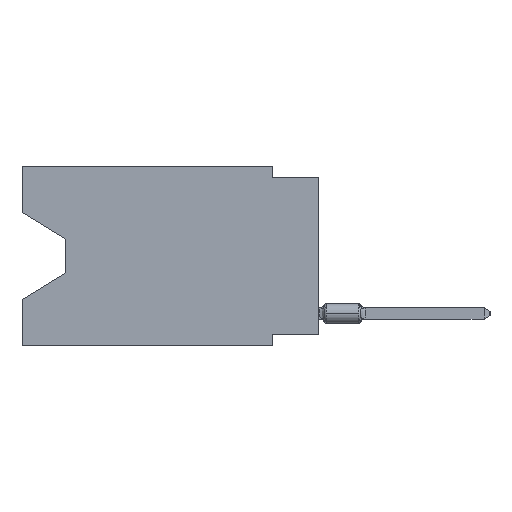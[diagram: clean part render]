
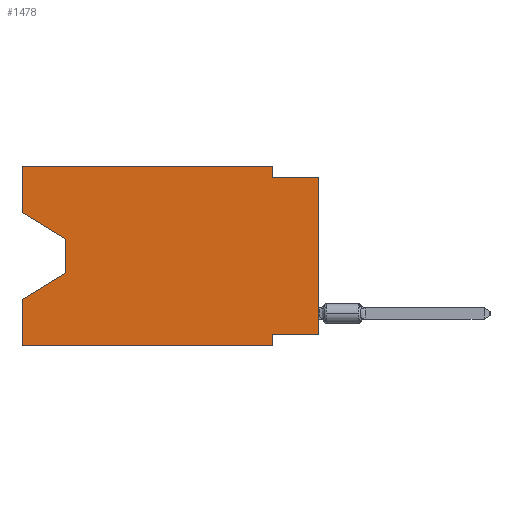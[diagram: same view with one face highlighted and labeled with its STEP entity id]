
A CAD part, left-side view. The second image highlights one B-rep face of the part: STEP entity #1478.
In plain terms, the highlighted planar face has unit normal (-1, 0, 0).
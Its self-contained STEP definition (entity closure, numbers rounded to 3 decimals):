
#391 = LINE ( 'NONE', #15423, #25079 ) ;
#925 = VERTEX_POINT ( 'NONE', #43220 ) ;
#1397 = CARTESIAN_POINT ( 'NONE',  ( 0., 16.383, -9.906 ) ) ;
#1478 = ADVANCED_FACE ( 'NONE', ( #54049 ), #12353, .F. ) ;
#2420 = DIRECTION ( 'NONE',  ( 1., 0., 0. ) ) ;
#3002 = DIRECTION ( 'NONE',  ( 0., 1., 0. ) ) ;
#3283 = VECTOR ( 'NONE', #44794, 1000. ) ;
#3491 = CARTESIAN_POINT ( 'NONE',  ( 0., 16.383, -9.906 ) ) ;
#3820 = LINE ( 'NONE', #13409, #64594 ) ;
#4241 = LINE ( 'NONE', #20308, #49185 ) ;
#4481 = VERTEX_POINT ( 'NONE', #1397 ) ;
#6366 = EDGE_CURVE ( 'NONE', #21469, #45907, #39562, .T. ) ;
#7596 = VERTEX_POINT ( 'NONE', #45051 ) ;
#8268 = AXIS2_PLACEMENT_3D ( 'NONE', #65319, #2420, #44143 ) ;
#8610 = VECTOR ( 'NONE', #54688, 1000. ) ;
#8970 = VECTOR ( 'NONE', #66699, 1000. ) ;
#8977 = EDGE_CURVE ( 'NONE', #925, #44547, #14672, .T. ) ;
#10274 = CARTESIAN_POINT ( 'NONE',  ( 0., 0., 0. ) ) ;
#11287 = LINE ( 'NONE', #10274, #15699 ) ;
#12353 = PLANE ( 'NONE',  #8268 ) ;
#13236 = VERTEX_POINT ( 'NONE', #47078 ) ;
#13409 = CARTESIAN_POINT ( 'NONE',  ( 0., 0., -0.635 ) ) ;
#14345 = CARTESIAN_POINT ( 'NONE',  ( 0., 13.97, -5.893 ) ) ;
#14672 = LINE ( 'NONE', #14345, #36406 ) ;
#14754 = CARTESIAN_POINT ( 'NONE',  ( 0., 13.97, -4.013 ) ) ;
#14878 = LINE ( 'NONE', #51452, #41210 ) ;
#15130 = ORIENTED_EDGE ( 'NONE', *, *, #55828, .T. ) ;
#15323 = ORIENTED_EDGE ( 'NONE', *, *, #56338, .F. ) ;
#15423 = CARTESIAN_POINT ( 'NONE',  ( 0., 13.97, -4.013 ) ) ;
#15699 = VECTOR ( 'NONE', #51976, 1000. ) ;
#16306 = VECTOR ( 'NONE', #29139, 1000. ) ;
#19307 = ORIENTED_EDGE ( 'NONE', *, *, #53118, .F. ) ;
#19395 = ORIENTED_EDGE ( 'NONE', *, *, #33960, .T. ) ;
#20308 = CARTESIAN_POINT ( 'NONE',  ( 0., 16.383, 0. ) ) ;
#20955 = ORIENTED_EDGE ( 'NONE', *, *, #58679, .F. ) ;
#21469 = VERTEX_POINT ( 'NONE', #47541 ) ;
#21693 = CARTESIAN_POINT ( 'NONE',  ( 0., 16.383, -7.36 ) ) ;
#22912 = CARTESIAN_POINT ( 'NONE',  ( 0., 16.383, 0. ) ) ;
#24276 = VERTEX_POINT ( 'NONE', #60544 ) ;
#25001 = LINE ( 'NONE', #3491, #16306 ) ;
#25079 = VECTOR ( 'NONE', #37634, 1000. ) ;
#26048 = ORIENTED_EDGE ( 'NONE', *, *, #28337, .F. ) ;
#27658 = ORIENTED_EDGE ( 'NONE', *, *, #63083, .T. ) ;
#28337 = EDGE_CURVE ( 'NONE', #13236, #43127, #49872, .T. ) ;
#29139 = DIRECTION ( 'NONE',  ( 0., -1., 0. ) ) ;
#30065 = DIRECTION ( 'NONE',  ( 0., 0.855, -0.519 ) ) ;
#33960 = EDGE_CURVE ( 'NONE', #13236, #54102, #14878, .T. ) ;
#34176 = CARTESIAN_POINT ( 'NONE',  ( 0., 2.54, -9.906 ) ) ;
#34948 = VERTEX_POINT ( 'NONE', #53314 ) ;
#36406 = VECTOR ( 'NONE', #30065, 1000. ) ;
#36752 = EDGE_LOOP ( 'NONE', ( #19395, #58672, #62324, #61145, #15130, #15323, #44596, #27658, #20955, #43640, #19307, #26048 ) ) ;
#37036 = VECTOR ( 'NONE', #3002, 1000. ) ;
#37634 = DIRECTION ( 'NONE',  ( 0., 0., -1. ) ) ;
#39562 = LINE ( 'NONE', #65878, #37036 ) ;
#41206 = DIRECTION ( 'NONE',  ( 0., -0.855, -0.519 ) ) ;
#41210 = VECTOR ( 'NONE', #41206, 1000. ) ;
#42430 = LINE ( 'NONE', #22912, #8610 ) ;
#42773 = CARTESIAN_POINT ( 'NONE',  ( 0., 2.54, -9.271 ) ) ;
#43127 = VERTEX_POINT ( 'NONE', #62383 ) ;
#43220 = CARTESIAN_POINT ( 'NONE',  ( 0., 13.97, -5.893 ) ) ;
#43308 = VECTOR ( 'NONE', #54653, 1000. ) ;
#43640 = ORIENTED_EDGE ( 'NONE', *, *, #49912, .F. ) ;
#44143 = DIRECTION ( 'NONE',  ( 0., 0., -1. ) ) ;
#44532 = DIRECTION ( 'NONE',  ( 0., -1., 0. ) ) ;
#44547 = VERTEX_POINT ( 'NONE', #21693 ) ;
#44596 = ORIENTED_EDGE ( 'NONE', *, *, #6366, .F. ) ;
#44794 = DIRECTION ( 'NONE',  ( 0., 0., -1. ) ) ;
#45051 = CARTESIAN_POINT ( 'NONE',  ( 0., 2.54, 0. ) ) ;
#45907 = VERTEX_POINT ( 'NONE', #42773 ) ;
#45944 = EDGE_CURVE ( 'NONE', #54102, #925, #391, .T. ) ;
#47078 = CARTESIAN_POINT ( 'NONE',  ( 0., 16.383, -2.546 ) ) ;
#47541 = CARTESIAN_POINT ( 'NONE',  ( 0., 0., -9.271 ) ) ;
#48787 = EDGE_CURVE ( 'NONE', #4481, #44547, #4241, .T. ) ;
#49185 = VECTOR ( 'NONE', #51405, 1000. ) ;
#49872 = LINE ( 'NONE', #61123, #43308 ) ;
#49912 = EDGE_CURVE ( 'NONE', #7596, #34948, #55776, .T. ) ;
#51405 = DIRECTION ( 'NONE',  ( 0., 0., 1. ) ) ;
#51452 = CARTESIAN_POINT ( 'NONE',  ( 0., 16.383, -2.546 ) ) ;
#51976 = DIRECTION ( 'NONE',  ( 0., 0., 1. ) ) ;
#53118 = EDGE_CURVE ( 'NONE', #43127, #7596, #42430, .T. ) ;
#53314 = CARTESIAN_POINT ( 'NONE',  ( 0., 2.54, -0.635 ) ) ;
#54049 = FACE_OUTER_BOUND ( 'NONE', #36752, .T. ) ;
#54102 = VERTEX_POINT ( 'NONE', #14754 ) ;
#54653 = DIRECTION ( 'NONE',  ( 0., 0., 1. ) ) ;
#54688 = DIRECTION ( 'NONE',  ( 0., -1., 0. ) ) ;
#55776 = LINE ( 'NONE', #61909, #8970 ) ;
#55828 = EDGE_CURVE ( 'NONE', #4481, #24276, #25001, .T. ) ;
#56338 = EDGE_CURVE ( 'NONE', #45907, #24276, #60163, .T. ) ;
#57040 = VERTEX_POINT ( 'NONE', #59311 ) ;
#58672 = ORIENTED_EDGE ( 'NONE', *, *, #45944, .T. ) ;
#58679 = EDGE_CURVE ( 'NONE', #34948, #57040, #3820, .T. ) ;
#59311 = CARTESIAN_POINT ( 'NONE',  ( 0., 0., -0.635 ) ) ;
#60163 = LINE ( 'NONE', #34176, #3283 ) ;
#60544 = CARTESIAN_POINT ( 'NONE',  ( 0., 2.54, -9.906 ) ) ;
#61123 = CARTESIAN_POINT ( 'NONE',  ( 0., 16.383, 0. ) ) ;
#61145 = ORIENTED_EDGE ( 'NONE', *, *, #48787, .F. ) ;
#61909 = CARTESIAN_POINT ( 'NONE',  ( 0., 2.54, 0. ) ) ;
#62324 = ORIENTED_EDGE ( 'NONE', *, *, #8977, .T. ) ;
#62383 = CARTESIAN_POINT ( 'NONE',  ( 0., 16.383, 0. ) ) ;
#63083 = EDGE_CURVE ( 'NONE', #21469, #57040, #11287, .T. ) ;
#64594 = VECTOR ( 'NONE', #44532, 1000. ) ;
#65319 = CARTESIAN_POINT ( 'NONE',  ( 0., 16.383, 0. ) ) ;
#65878 = CARTESIAN_POINT ( 'NONE',  ( 0., 0., -9.271 ) ) ;
#66699 = DIRECTION ( 'NONE',  ( 0., 0., -1. ) ) ;
